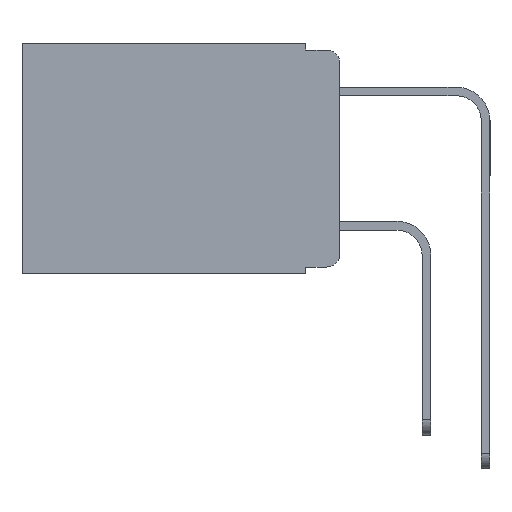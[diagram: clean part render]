
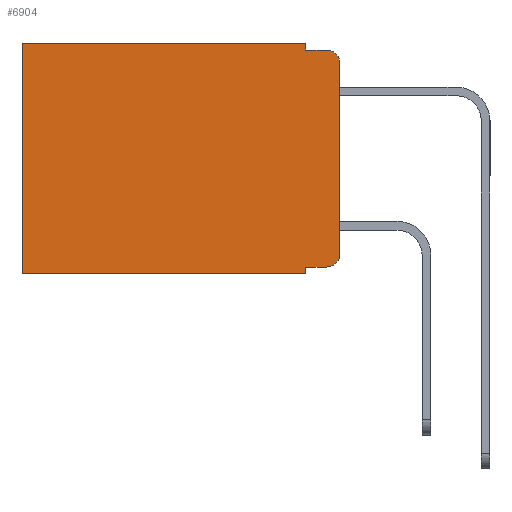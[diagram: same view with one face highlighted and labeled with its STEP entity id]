
A CAD part, left-side view. The second image highlights one B-rep face of the part: STEP entity #6904.
In plain terms, the highlighted planar face has unit normal (-1, 0, 0).
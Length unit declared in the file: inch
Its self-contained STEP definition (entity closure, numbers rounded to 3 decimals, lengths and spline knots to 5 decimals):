
#456 = EDGE_CURVE ( 'NONE', #15211, #16667, #15344, .T. ) ;
#507 = VERTEX_POINT ( 'NONE', #10480 ) ;
#700 = CIRCLE ( 'NONE', #17856, 0.02 ) ;
#916 = DIRECTION ( 'NONE',  ( 0., 0., -1. ) ) ;
#945 = EDGE_CURVE ( 'NONE', #22499, #16667, #19969, .T. ) ;
#1477 = CARTESIAN_POINT ( 'NONE',  ( 0.298, 0.051, -0.333 ) ) ;
#1644 = DIRECTION ( 'NONE',  ( 0., -1., 0. ) ) ;
#1882 = VERTEX_POINT ( 'NONE', #12102 ) ;
#1904 = DIRECTION ( 'NONE',  ( 0., 0., -1. ) ) ;
#2691 = CARTESIAN_POINT ( 'NONE',  ( 0.298, 0.02, -0.03 ) ) ;
#3328 = DIRECTION ( 'NONE',  ( 0., 0., -1. ) ) ;
#4329 = ORIENTED_EDGE ( 'NONE', *, *, #9863, .T. ) ;
#4556 = EDGE_CURVE ( 'NONE', #12068, #16100, #700, .T. ) ;
#4558 = LINE ( 'NONE', #18926, #17233 ) ;
#4610 = CARTESIAN_POINT ( 'NONE',  ( 0.298, 0.02, -0.333 ) ) ;
#4665 = LINE ( 'NONE', #16215, #22530 ) ;
#4679 = CARTESIAN_POINT ( 'NONE',  ( 0.298, 0., 0. ) ) ;
#4784 = VECTOR ( 'NONE', #1904, 39.37008 ) ;
#4928 = ORIENTED_EDGE ( 'NONE', *, *, #7210, .T. ) ;
#5034 = CARTESIAN_POINT ( 'NONE',  ( 0.298, 0., 0. ) ) ;
#5065 = ORIENTED_EDGE ( 'NONE', *, *, #18592, .F. ) ;
#5269 = VECTOR ( 'NONE', #5993, 39.37008 ) ;
#5795 = LINE ( 'NONE', #13791, #18937 ) ;
#5853 = ORIENTED_EDGE ( 'NONE', *, *, #945, .F. ) ;
#5993 = DIRECTION ( 'NONE',  ( 0., 0., -1. ) ) ;
#6597 = CARTESIAN_POINT ( 'NONE',  ( 0.298, 0.051, -0.01 ) ) ;
#6635 = VERTEX_POINT ( 'NONE', #7813 ) ;
#6876 = DIRECTION ( 'NONE',  ( 1., 0., 0. ) ) ;
#6904 = ADVANCED_FACE ( 'NONE', ( #14637 ), #20442, .F. ) ;
#7210 = EDGE_CURVE ( 'NONE', #507, #15857, #4665, .T. ) ;
#7392 = AXIS2_PLACEMENT_3D ( 'NONE', #2691, #11462, #16930 ) ;
#7589 = LINE ( 'NONE', #4679, #12603 ) ;
#7625 = EDGE_CURVE ( 'NONE', #14037, #6635, #5795, .T. ) ;
#7645 = ORIENTED_EDGE ( 'NONE', *, *, #456, .T. ) ;
#7787 = DIRECTION ( 'NONE',  ( 0., 1., 0. ) ) ;
#7813 = CARTESIAN_POINT ( 'NONE',  ( 0.298, 0.051, -0.343 ) ) ;
#7949 = ORIENTED_EDGE ( 'NONE', *, *, #10159, .F. ) ;
#8748 = VECTOR ( 'NONE', #1644, 39.37008 ) ;
#8850 = CARTESIAN_POINT ( 'NONE',  ( 0.298, 0.02, -0.313 ) ) ;
#9863 = EDGE_CURVE ( 'NONE', #15857, #1882, #18536, .T. ) ;
#10159 = EDGE_CURVE ( 'NONE', #15211, #16100, #7589, .T. ) ;
#10161 = CARTESIAN_POINT ( 'NONE',  ( 0.298, 0., -0.03 ) ) ;
#10480 = CARTESIAN_POINT ( 'NONE',  ( 0.298, 0.051, 0. ) ) ;
#10494 = CARTESIAN_POINT ( 'NONE',  ( 0.298, 0.473, 0. ) ) ;
#11462 = DIRECTION ( 'NONE',  ( -1., 0., 0. ) ) ;
#11741 = AXIS2_PLACEMENT_3D ( 'NONE', #5034, #6876, #18815 ) ;
#12068 = VERTEX_POINT ( 'NONE', #4610 ) ;
#12102 = CARTESIAN_POINT ( 'NONE',  ( 0.298, 0.473, -0.343 ) ) ;
#12253 = CARTESIAN_POINT ( 'NONE',  ( 0.298, 0.051, -0.333 ) ) ;
#12603 = VECTOR ( 'NONE', #916, 39.37008 ) ;
#13204 = LINE ( 'NONE', #12253, #8748 ) ;
#13295 = DIRECTION ( 'NONE',  ( -1., 0., 0. ) ) ;
#13706 = DIRECTION ( 'NONE',  ( 0., 1., 0. ) ) ;
#13791 = CARTESIAN_POINT ( 'NONE',  ( 0.298, 0.051, 0. ) ) ;
#14020 = EDGE_CURVE ( 'NONE', #6635, #1882, #4558, .T. ) ;
#14037 = VERTEX_POINT ( 'NONE', #1477 ) ;
#14373 = DIRECTION ( 'NONE',  ( 0., 0., -1. ) ) ;
#14637 = FACE_OUTER_BOUND ( 'NONE', #20294, .T. ) ;
#15211 = VERTEX_POINT ( 'NONE', #10161 ) ;
#15323 = VECTOR ( 'NONE', #18765, 39.37008 ) ;
#15344 = CIRCLE ( 'NONE', #7392, 0.02 ) ;
#15857 = VERTEX_POINT ( 'NONE', #20557 ) ;
#15882 = CARTESIAN_POINT ( 'NONE',  ( 0.298, 0., -0.313 ) ) ;
#16100 = VERTEX_POINT ( 'NONE', #15882 ) ;
#16215 = CARTESIAN_POINT ( 'NONE',  ( 0.298, 0., 0. ) ) ;
#16667 = VERTEX_POINT ( 'NONE', #21131 ) ;
#16930 = DIRECTION ( 'NONE',  ( 0., 0., -1. ) ) ;
#17233 = VECTOR ( 'NONE', #13706, 39.37008 ) ;
#17856 = AXIS2_PLACEMENT_3D ( 'NONE', #8850, #13295, #14373 ) ;
#17864 = ORIENTED_EDGE ( 'NONE', *, *, #14020, .F. ) ;
#18162 = ORIENTED_EDGE ( 'NONE', *, *, #4556, .T. ) ;
#18536 = LINE ( 'NONE', #10494, #4784 ) ;
#18592 = EDGE_CURVE ( 'NONE', #507, #22499, #19000, .T. ) ;
#18765 = DIRECTION ( 'NONE',  ( 0., -1., 0. ) ) ;
#18815 = DIRECTION ( 'NONE',  ( 0., 0., -1. ) ) ;
#18926 = CARTESIAN_POINT ( 'NONE',  ( 0.298, 0., -0.343 ) ) ;
#18937 = VECTOR ( 'NONE', #3328, 39.37008 ) ;
#19000 = LINE ( 'NONE', #19725, #5269 ) ;
#19725 = CARTESIAN_POINT ( 'NONE',  ( 0.298, 0.051, 0. ) ) ;
#19969 = LINE ( 'NONE', #6597, #15323 ) ;
#20294 = EDGE_LOOP ( 'NONE', ( #7949, #7645, #5853, #5065, #4928, #4329, #17864, #20661, #22054, #18162 ) ) ;
#20442 = PLANE ( 'NONE',  #11741 ) ;
#20557 = CARTESIAN_POINT ( 'NONE',  ( 0.298, 0.473, 0. ) ) ;
#20661 = ORIENTED_EDGE ( 'NONE', *, *, #7625, .F. ) ;
#21106 = CARTESIAN_POINT ( 'NONE',  ( 0.298, 0.051, -0.01 ) ) ;
#21131 = CARTESIAN_POINT ( 'NONE',  ( 0.298, 0.02, -0.01 ) ) ;
#21242 = EDGE_CURVE ( 'NONE', #14037, #12068, #13204, .T. ) ;
#22054 = ORIENTED_EDGE ( 'NONE', *, *, #21242, .T. ) ;
#22499 = VERTEX_POINT ( 'NONE', #21106 ) ;
#22530 = VECTOR ( 'NONE', #7787, 39.37008 ) ;
